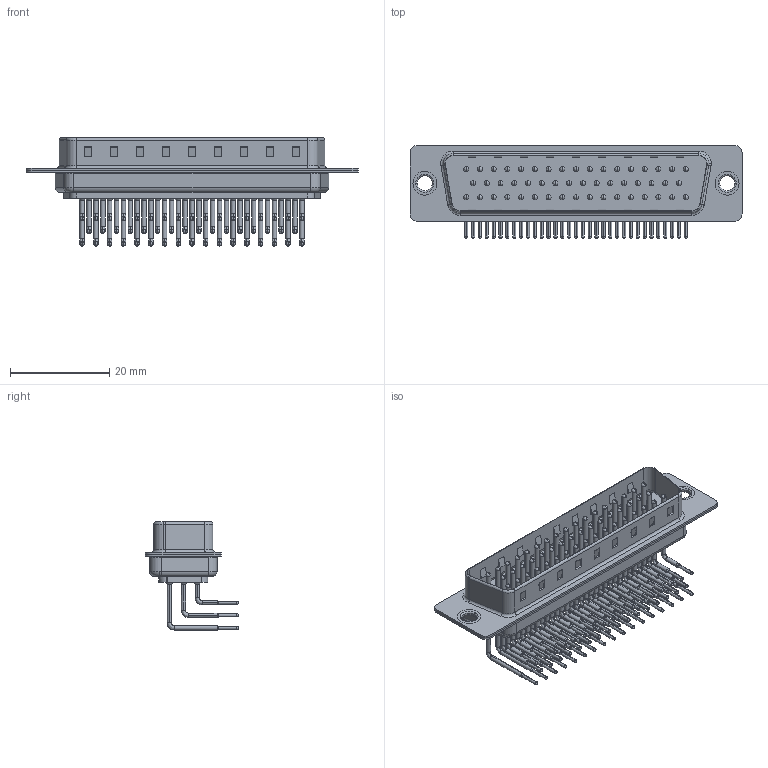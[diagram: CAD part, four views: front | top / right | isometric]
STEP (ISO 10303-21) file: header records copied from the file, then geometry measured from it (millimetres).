
FILE_DESCRIPTION (( 'STEP AP203' ), '1' );
FILE_NAME ('629-M50-340-LT1.STEP', '2018-09-26T00:42:25', ( '' ), ( '' ), 'SwSTEP 2.0', 'SolidWorks 2016', '' );
FILE_SCHEMA (( 'CONFIG_CONTROL_DESIGN' ));
Length unit declared in the file: millimetre
Products named in the file (8): 629M Contact Row 1_50 Contacts; 629M Contact Row 2_50 Contacts; 629M Contact Row 3; 629M Thru Hole Rivet; 629-M50-340-LT1; 629M Housing_50 Contacts; 629M Shell Front_50 Contacts; 629M Shell Rear_50 Contacts
Assembly tree (55 placements, depth 2):
  629-M50-340-LT1
    629M Housing_50 Contacts
    629M Shell Front_50 Contacts
    629M Shell Rear_50 Contacts
    629M Contact Row 1_50 Contacts  x17
    629M Contact Row 2_50 Contacts  x16
    629M Contact Row 3  x17
    629M Thru Hole Rivet  x2
Bounding box: 67 x 18.8 x 21.83 mm (x, y, z)
Volume: 4911.6 mm3; surface area: 12744 mm2
Topology: 55 solids, 55 shells, 5886 faces, 16509 edges, 10744 vertices
Faces by surface type: plane 3403, cylinder 1925, bspline 300, cone 200, torus 58
Entity records: 35304 total; most frequent: DIRECTION 6035, CARTESIAN_POINT 5923, ORIENTED_EDGE 5402, EDGE_CURVE 2701, AXIS2_PLACEMENT_3D 2237, VERTEX_POINT 1758, LINE 1561, VECTOR 1561
